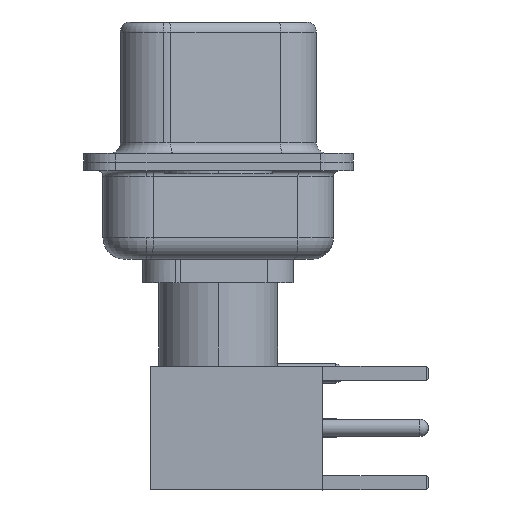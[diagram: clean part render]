
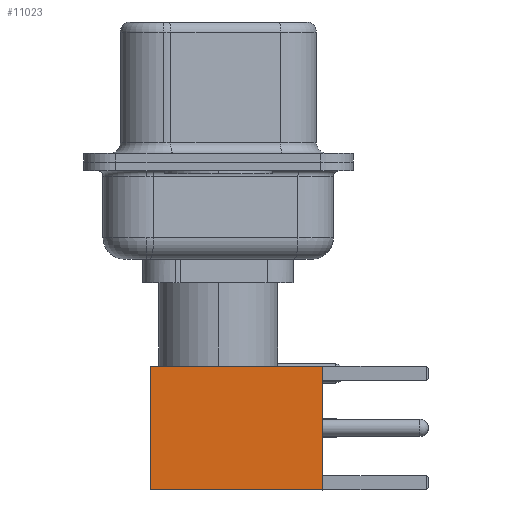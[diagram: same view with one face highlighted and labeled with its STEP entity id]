
A CAD part, left-side view. The second image highlights one B-rep face of the part: STEP entity #11023.
In plain terms, the highlighted face is planar.
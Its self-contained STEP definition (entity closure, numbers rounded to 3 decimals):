
#749 = CARTESIAN_POINT ( 'NONE',  ( -2.875, 2.875, 0. ) ) ;
#1042 = DIRECTION ( 'NONE',  ( 0., 0., -1. ) ) ;
#2644 = DIRECTION ( 'NONE',  ( 0., 0., 1. ) ) ;
#3469 = VERTEX_POINT ( 'NONE', #6498 ) ;
#4637 = PLANE ( 'NONE',  #12669 ) ;
#4850 = LINE ( 'NONE', #5117, #11695 ) ;
#5117 = CARTESIAN_POINT ( 'NONE',  ( 0., 2.875, 0. ) ) ;
#5162 = LINE ( 'NONE', #15616, #25277 ) ;
#5425 = VERTEX_POINT ( 'NONE', #23539 ) ;
#6498 = CARTESIAN_POINT ( 'NONE',  ( -2.875, 2.875, 0. ) ) ;
#6797 = ORIENTED_EDGE ( 'NONE', *, *, #15677, .T. ) ;
#6814 = CARTESIAN_POINT ( 'NONE',  ( -2.875, 2.875, 8. ) ) ;
#7031 = ORIENTED_EDGE ( 'NONE', *, *, #26341, .F. ) ;
#7863 = EDGE_CURVE ( 'NONE', #22280, #3469, #4850, .T. ) ;
#8630 = DIRECTION ( 'NONE',  ( -1., 0., 0. ) ) ;
#10464 = ORIENTED_EDGE ( 'NONE', *, *, #7863, .T. ) ;
#10769 = LINE ( 'NONE', #18806, #12871 ) ;
#10895 = DIRECTION ( 'NONE',  ( 0., 0., -1. ) ) ;
#11023 = ADVANCED_FACE ( 'NONE', ( #14816 ), #4637, .T. ) ;
#11695 = VECTOR ( 'NONE', #15422, 1000. ) ;
#11755 = CARTESIAN_POINT ( 'NONE',  ( 2.875, 2.875, 0. ) ) ;
#12669 = AXIS2_PLACEMENT_3D ( 'NONE', #12797, #20930, #2644 ) ;
#12797 = CARTESIAN_POINT ( 'NONE',  ( 2.875, 2.875, 0. ) ) ;
#12871 = VECTOR ( 'NONE', #8630, 1000. ) ;
#14816 = FACE_OUTER_BOUND ( 'NONE', #20571, .T. ) ;
#15422 = DIRECTION ( 'NONE',  ( -1., 0., 0. ) ) ;
#15616 = CARTESIAN_POINT ( 'NONE',  ( 2.875, 2.875, 0. ) ) ;
#15677 = EDGE_CURVE ( 'NONE', #5425, #22280, #5162, .T. ) ;
#18806 = CARTESIAN_POINT ( 'NONE',  ( 0., 2.875, 8. ) ) ;
#20142 = VECTOR ( 'NONE', #10895, 1000. ) ;
#20571 = EDGE_LOOP ( 'NONE', ( #6797, #10464, #21962, #7031 ) ) ;
#20930 = DIRECTION ( 'NONE',  ( 0., 1., 0. ) ) ;
#21962 = ORIENTED_EDGE ( 'NONE', *, *, #25090, .F. ) ;
#21976 = VERTEX_POINT ( 'NONE', #6814 ) ;
#22280 = VERTEX_POINT ( 'NONE', #11755 ) ;
#23539 = CARTESIAN_POINT ( 'NONE',  ( 2.875, 2.875, 8. ) ) ;
#25090 = EDGE_CURVE ( 'NONE', #21976, #3469, #25168, .T. ) ;
#25168 = LINE ( 'NONE', #749, #20142 ) ;
#25277 = VECTOR ( 'NONE', #1042, 1000. ) ;
#26341 = EDGE_CURVE ( 'NONE', #5425, #21976, #10769, .T. ) ;
